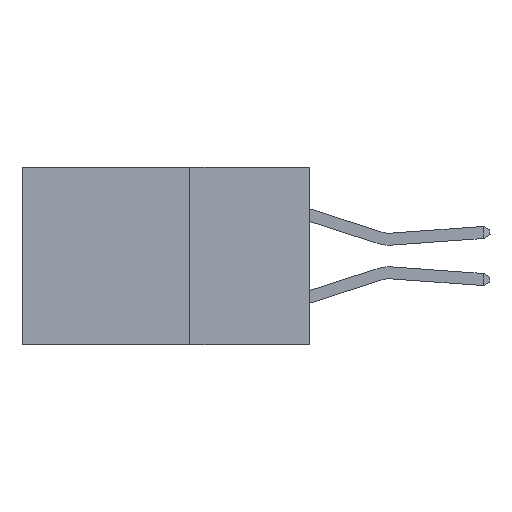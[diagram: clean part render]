
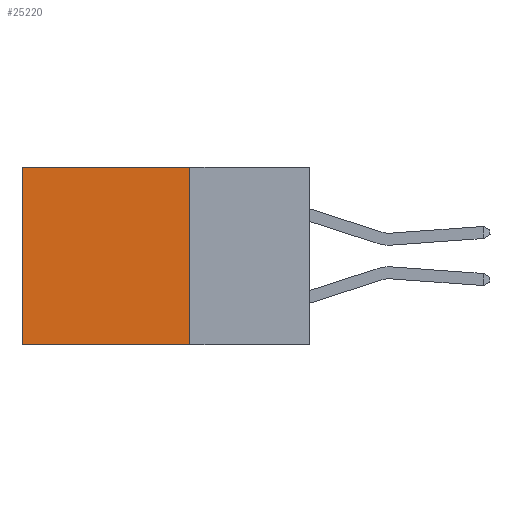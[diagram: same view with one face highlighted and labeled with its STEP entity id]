
A CAD part, left-side view. The second image highlights one B-rep face of the part: STEP entity #25220.
In plain terms, the highlighted planar face has unit normal (-1, 0, 0).
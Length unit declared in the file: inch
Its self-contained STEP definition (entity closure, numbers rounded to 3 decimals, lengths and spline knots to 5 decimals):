
#8 = EDGE_CURVE ( 'NONE', #22395, #11965, #21228, .T. ) ;
#189 = DIRECTION ( 'NONE',  ( 0., 0., -1. ) ) ;
#492 = VERTEX_POINT ( 'NONE', #21053 ) ;
#910 = DIRECTION ( 'NONE',  ( 1., 0., 0. ) ) ;
#1060 = VECTOR ( 'NONE', #189, 39.37008 ) ;
#1157 = EDGE_CURVE ( 'NONE', #11965, #492, #18234, .T. ) ;
#1578 = EDGE_LOOP ( 'NONE', ( #16400, #7114, #7075, #2231 ) ) ;
#2231 = ORIENTED_EDGE ( 'NONE', *, *, #7651, .T. ) ;
#5184 = DIRECTION ( 'NONE',  ( 0., 0., -1. ) ) ;
#5831 = CARTESIAN_POINT ( 'NONE',  ( 0.2615, 0.25, -0.37 ) ) ;
#7075 = ORIENTED_EDGE ( 'NONE', *, *, #8, .F. ) ;
#7114 = ORIENTED_EDGE ( 'NONE', *, *, #1157, .F. ) ;
#7651 = EDGE_CURVE ( 'NONE', #22395, #14330, #8822, .T. ) ;
#7734 = VECTOR ( 'NONE', #16527, 39.37008 ) ;
#8822 = LINE ( 'NONE', #21008, #18757 ) ;
#8848 = EDGE_CURVE ( 'NONE', #14330, #492, #9894, .T. ) ;
#9894 = LINE ( 'NONE', #17775, #1060 ) ;
#11114 = CARTESIAN_POINT ( 'NONE',  ( 0.2615, 0.25, -0.37 ) ) ;
#11158 = DIRECTION ( 'NONE',  ( 0., 1., 0. ) ) ;
#11664 = AXIS2_PLACEMENT_3D ( 'NONE', #11114, #910, #5184 ) ;
#11715 = CARTESIAN_POINT ( 'NONE',  ( 0.2615, 0.25, -0.37 ) ) ;
#11796 = VECTOR ( 'NONE', #21606, 39.37008 ) ;
#11965 = VERTEX_POINT ( 'NONE', #11715 ) ;
#14330 = VERTEX_POINT ( 'NONE', #14369 ) ;
#14369 = CARTESIAN_POINT ( 'NONE',  ( 0.2615, 0.6, 0. ) ) ;
#14467 = CARTESIAN_POINT ( 'NONE',  ( 0.2615, 0.25, -0.37 ) ) ;
#14860 = PLANE ( 'NONE',  #11664 ) ;
#16400 = ORIENTED_EDGE ( 'NONE', *, *, #8848, .T. ) ;
#16527 = DIRECTION ( 'NONE',  ( 0., 1., 0. ) ) ;
#17173 = FACE_OUTER_BOUND ( 'NONE', #1578, .T. ) ;
#17775 = CARTESIAN_POINT ( 'NONE',  ( 0.2615, 0.6, -0.37 ) ) ;
#18234 = LINE ( 'NONE', #14467, #7734 ) ;
#18757 = VECTOR ( 'NONE', #11158, 39.37008 ) ;
#21008 = CARTESIAN_POINT ( 'NONE',  ( 0.2615, 0.25, 0. ) ) ;
#21053 = CARTESIAN_POINT ( 'NONE',  ( 0.2615, 0.6, -0.37 ) ) ;
#21228 = LINE ( 'NONE', #5831, #11796 ) ;
#21606 = DIRECTION ( 'NONE',  ( 0., 0., -1. ) ) ;
#22395 = VERTEX_POINT ( 'NONE', #24375 ) ;
#24375 = CARTESIAN_POINT ( 'NONE',  ( 0.2615, 0.25, 0. ) ) ;
#25220 = ADVANCED_FACE ( 'NONE', ( #17173 ), #14860, .F. ) ;
